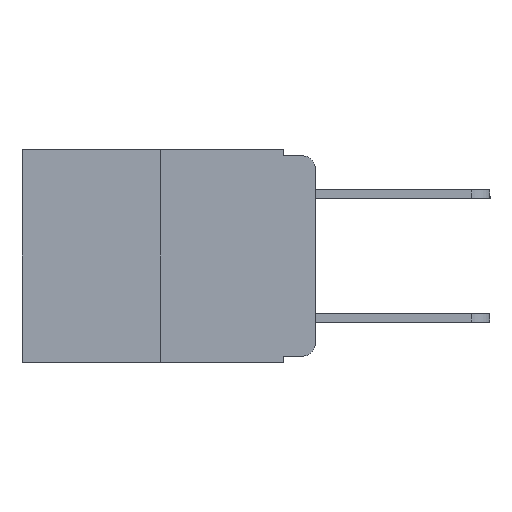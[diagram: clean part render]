
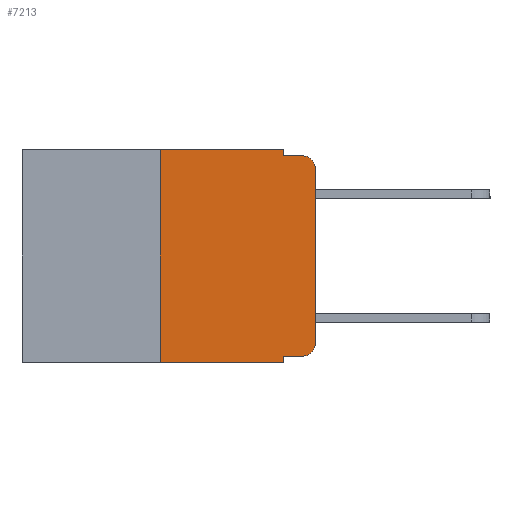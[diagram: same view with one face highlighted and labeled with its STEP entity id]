
A CAD part, left-side view. The second image highlights one B-rep face of the part: STEP entity #7213.
In plain terms, the highlighted planar face has unit normal (-1, 0, 0).
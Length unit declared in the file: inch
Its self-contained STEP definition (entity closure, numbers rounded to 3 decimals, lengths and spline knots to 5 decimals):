
#199 = VERTEX_POINT ( 'NONE', #4011 ) ;
#216 = CARTESIAN_POINT ( 'NONE',  ( 0., 0.473, 0. ) ) ;
#234 = CARTESIAN_POINT ( 'NONE',  ( 0., 0.02, -0.03 ) ) ;
#284 = DIRECTION ( 'NONE',  ( 0., 0., -1. ) ) ;
#298 = DIRECTION ( 'NONE',  ( 0., 0., 1. ) ) ;
#328 = ORIENTED_EDGE ( 'NONE', *, *, #3633, .T. ) ;
#336 = ORIENTED_EDGE ( 'NONE', *, *, #4623, .F. ) ;
#453 = VERTEX_POINT ( 'NONE', #2755 ) ;
#472 = ORIENTED_EDGE ( 'NONE', *, *, #6256, .F. ) ;
#580 = ORIENTED_EDGE ( 'NONE', *, *, #8160, .F. ) ;
#593 = VERTEX_POINT ( 'NONE', #5707 ) ;
#806 = DIRECTION ( 'NONE',  ( -1., 0., 0. ) ) ;
#819 = VERTEX_POINT ( 'NONE', #7087 ) ;
#1191 = CARTESIAN_POINT ( 'NONE',  ( 0., 0.051, -0.333 ) ) ;
#1214 = DIRECTION ( 'NONE',  ( 0., 0., -1. ) ) ;
#1458 = ORIENTED_EDGE ( 'NONE', *, *, #6242, .T. ) ;
#1469 = ORIENTED_EDGE ( 'NONE', *, *, #6225, .T. ) ;
#1690 = VERTEX_POINT ( 'NONE', #1191 ) ;
#1854 = VECTOR ( 'NONE', #7359, 39.37008 ) ;
#1916 = VERTEX_POINT ( 'NONE', #6950 ) ;
#2005 = DIRECTION ( 'NONE',  ( 0., -1., 0. ) ) ;
#2211 = AXIS2_PLACEMENT_3D ( 'NONE', #6025, #806, #6847 ) ;
#2319 = CARTESIAN_POINT ( 'NONE',  ( 0., 0., -0.03 ) ) ;
#2477 = CIRCLE ( 'NONE', #8024, 0.02 ) ;
#2632 = DIRECTION ( 'NONE',  ( 0., 0., 1. ) ) ;
#2696 = DIRECTION ( 'NONE',  ( 0., 0., -1. ) ) ;
#2755 = CARTESIAN_POINT ( 'NONE',  ( 0., 0.02, -0.01 ) ) ;
#2766 = ORIENTED_EDGE ( 'NONE', *, *, #6063, .T. ) ;
#2931 = ORIENTED_EDGE ( 'NONE', *, *, #6258, .F. ) ;
#3074 = VECTOR ( 'NONE', #2005, 39.37008 ) ;
#3165 = VECTOR ( 'NONE', #2632, 39.37008 ) ;
#3175 = VECTOR ( 'NONE', #298, 39.37008 ) ;
#3218 = EDGE_LOOP ( 'NONE', ( #2766, #3906, #580, #9833, #336, #2931, #328, #472, #1458, #1469 ) ) ;
#3229 = DIRECTION ( 'NONE',  ( 0., -1., 0. ) ) ;
#3439 = CARTESIAN_POINT ( 'NONE',  ( 0., 0.051, 0. ) ) ;
#3442 = LINE ( 'NONE', #3439, #7733 ) ;
#3633 = EDGE_CURVE ( 'NONE', #5156, #1916, #8340, .T. ) ;
#3778 = CARTESIAN_POINT ( 'NONE',  ( 0., 0.473, -0.343 ) ) ;
#3906 = ORIENTED_EDGE ( 'NONE', *, *, #9430, .T. ) ;
#4011 = CARTESIAN_POINT ( 'NONE',  ( 0., 0., -0.313 ) ) ;
#4508 = VERTEX_POINT ( 'NONE', #9657 ) ;
#4572 = VECTOR ( 'NONE', #2696, 39.37008 ) ;
#4623 = EDGE_CURVE ( 'NONE', #4508, #819, #9620, .T. ) ;
#4686 = PLANE ( 'NONE',  #10368 ) ;
#5073 = VERTEX_POINT ( 'NONE', #2319 ) ;
#5156 = VERTEX_POINT ( 'NONE', #5982 ) ;
#5204 = CARTESIAN_POINT ( 'NONE',  ( 0., 0.051, -0.333 ) ) ;
#5247 = CARTESIAN_POINT ( 'NONE',  ( 0., 0.25, 0. ) ) ;
#5248 = LINE ( 'NONE', #5588, #3175 ) ;
#5577 = DIRECTION ( 'NONE',  ( 1., 0., 0. ) ) ;
#5588 = CARTESIAN_POINT ( 'NONE',  ( 0., 0., 0. ) ) ;
#5690 = CARTESIAN_POINT ( 'NONE',  ( 0., 0.051, -0.01 ) ) ;
#5707 = CARTESIAN_POINT ( 'NONE',  ( 0., 0.051, -0.01 ) ) ;
#5982 = CARTESIAN_POINT ( 'NONE',  ( 0., 0.25, -0.343 ) ) ;
#6025 = CARTESIAN_POINT ( 'NONE',  ( 0., 0.02, -0.313 ) ) ;
#6063 = EDGE_CURVE ( 'NONE', #199, #5073, #5248, .T. ) ;
#6126 = VECTOR ( 'NONE', #3229, 39.37008 ) ;
#6225 = EDGE_CURVE ( 'NONE', #6948, #199, #8709, .T. ) ;
#6242 = EDGE_CURVE ( 'NONE', #1690, #6948, #8259, .T. ) ;
#6256 = EDGE_CURVE ( 'NONE', #1690, #1916, #3442, .T. ) ;
#6258 = EDGE_CURVE ( 'NONE', #5156, #4508, #9900, .T. ) ;
#6278 = EDGE_CURVE ( 'NONE', #819, #593, #8748, .T. ) ;
#6374 = DIRECTION ( 'NONE',  ( -1., 0., 0. ) ) ;
#6847 = DIRECTION ( 'NONE',  ( 0., 0., -1. ) ) ;
#6948 = VERTEX_POINT ( 'NONE', #10035 ) ;
#6950 = CARTESIAN_POINT ( 'NONE',  ( 0., 0.051, -0.343 ) ) ;
#7087 = CARTESIAN_POINT ( 'NONE',  ( 0., 0.051, 0. ) ) ;
#7213 = ADVANCED_FACE ( 'NONE', ( #10333 ), #4686, .F. ) ;
#7359 = DIRECTION ( 'NONE',  ( 0., -1., 0. ) ) ;
#7733 = VECTOR ( 'NONE', #7779, 39.37008 ) ;
#7743 = DIRECTION ( 'NONE',  ( 0., -1., 0. ) ) ;
#7779 = DIRECTION ( 'NONE',  ( 0., 0., -1. ) ) ;
#7996 = VECTOR ( 'NONE', #7743, 39.37008 ) ;
#8024 = AXIS2_PLACEMENT_3D ( 'NONE', #234, #6374, #1214 ) ;
#8160 = EDGE_CURVE ( 'NONE', #593, #453, #9028, .T. ) ;
#8259 = LINE ( 'NONE', #5204, #7996 ) ;
#8340 = LINE ( 'NONE', #3778, #6126 ) ;
#8709 = CIRCLE ( 'NONE', #2211, 0.02 ) ;
#8748 = LINE ( 'NONE', #9321, #4572 ) ;
#9028 = LINE ( 'NONE', #5690, #1854 ) ;
#9321 = CARTESIAN_POINT ( 'NONE',  ( 0., 0.051, 0. ) ) ;
#9430 = EDGE_CURVE ( 'NONE', #5073, #453, #2477, .T. ) ;
#9620 = LINE ( 'NONE', #216, #3074 ) ;
#9657 = CARTESIAN_POINT ( 'NONE',  ( 0., 0.25, 0. ) ) ;
#9833 = ORIENTED_EDGE ( 'NONE', *, *, #6278, .F. ) ;
#9900 = LINE ( 'NONE', #5247, #3165 ) ;
#10035 = CARTESIAN_POINT ( 'NONE',  ( 0., 0.02, -0.333 ) ) ;
#10187 = CARTESIAN_POINT ( 'NONE',  ( 0., 0.473, 0. ) ) ;
#10333 = FACE_OUTER_BOUND ( 'NONE', #3218, .T. ) ;
#10368 = AXIS2_PLACEMENT_3D ( 'NONE', #10187, #5577, #284 ) ;
